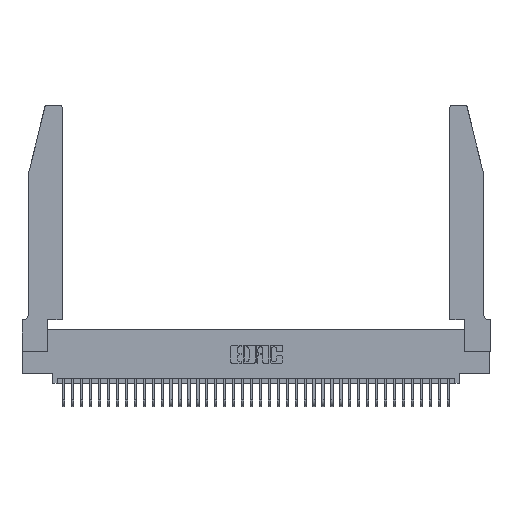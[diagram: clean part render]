
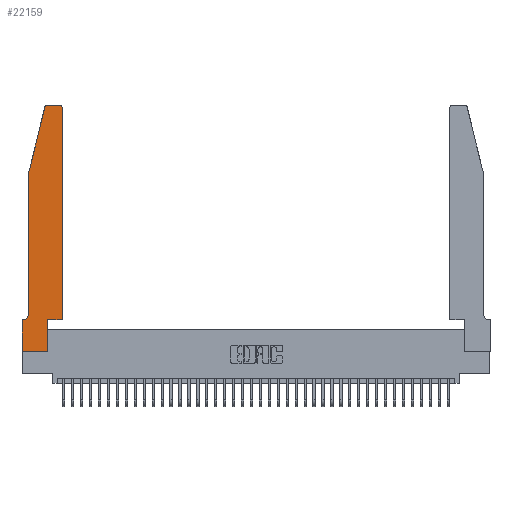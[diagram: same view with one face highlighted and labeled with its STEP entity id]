
A CAD part, top view. The second image highlights one B-rep face of the part: STEP entity #22159.
In plain terms, the highlighted planar face has unit normal (0, 0, 1).
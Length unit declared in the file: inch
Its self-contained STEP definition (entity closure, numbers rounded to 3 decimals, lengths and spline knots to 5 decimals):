
#625 = EDGE_CURVE ( 'NONE', #36127, #12795, #16288, .T. ) ;
#1551 = CARTESIAN_POINT ( 'NONE',  ( 0.4505, 0.35, 0.37 ) ) ;
#2278 = CARTESIAN_POINT ( 'NONE',  ( 0.4505, 2.72, 0.37 ) ) ;
#2791 = CIRCLE ( 'NONE', #31797, 0.03 ) ;
#3465 = EDGE_CURVE ( 'NONE', #24443, #10133, #4185, .T. ) ;
#3854 = CARTESIAN_POINT ( 'NONE',  ( 0., 0.35, 0.37 ) ) ;
#4185 = LINE ( 'NONE', #26175, #34276 ) ;
#4391 = VERTEX_POINT ( 'NONE', #27126 ) ;
#4457 = CARTESIAN_POINT ( 'NONE',  ( 0.4505, 0.35, 0.37 ) ) ;
#4560 = DIRECTION ( 'NONE',  ( 0., 1., 0. ) ) ;
#5130 = CARTESIAN_POINT ( 'NONE',  ( 0.4505, 0.35, 0.37 ) ) ;
#5226 = PLANE ( 'NONE',  #8894 ) ;
#5331 = VECTOR ( 'NONE', #26125, 39.37008 ) ;
#5971 = VECTOR ( 'NONE', #6633, 39.37008 ) ;
#6633 = DIRECTION ( 'NONE',  ( 0., -1., 0. ) ) ;
#6661 = VECTOR ( 'NONE', #24612, 39.37008 ) ;
#7060 = LINE ( 'NONE', #1551, #21715 ) ;
#7087 = CARTESIAN_POINT ( 'NONE',  ( 0.0055, 0.42, 0.37 ) ) ;
#7164 = CARTESIAN_POINT ( 'NONE',  ( 0.2865, 0.35, 0.37 ) ) ;
#7253 = ORIENTED_EDGE ( 'NONE', *, *, #16335, .T. ) ;
#7454 = VECTOR ( 'NONE', #10865, 39.37008 ) ;
#7785 = VERTEX_POINT ( 'NONE', #35398 ) ;
#8198 = DIRECTION ( 'NONE',  ( 1., 0., 0. ) ) ;
#8477 = CARTESIAN_POINT ( 'NONE',  ( 0.0755, 2., 0.37 ) ) ;
#8894 = AXIS2_PLACEMENT_3D ( 'NONE', #22671, #25734, #8198 ) ;
#8982 = VERTEX_POINT ( 'NONE', #23727 ) ;
#9680 = ORIENTED_EDGE ( 'NONE', *, *, #31655, .T. ) ;
#9687 = CARTESIAN_POINT ( 'NONE',  ( 0.4205, 2.72, 0.37 ) ) ;
#9703 = FACE_OUTER_BOUND ( 'NONE', #21059, .T. ) ;
#10053 = DIRECTION ( 'NONE',  ( -1., 0., 0. ) ) ;
#10133 = VERTEX_POINT ( 'NONE', #14189 ) ;
#10865 = DIRECTION ( 'NONE',  ( 1., 0., 0. ) ) ;
#11170 = ORIENTED_EDGE ( 'NONE', *, *, #29424, .T. ) ;
#11819 = ORIENTED_EDGE ( 'NONE', *, *, #21625, .T. ) ;
#12626 = DIRECTION ( 'NONE',  ( 1., 0., 0. ) ) ;
#12795 = VERTEX_POINT ( 'NONE', #3854 ) ;
#13586 = DIRECTION ( 'NONE',  ( 0., -1., 0. ) ) ;
#13634 = EDGE_CURVE ( 'NONE', #7785, #8982, #29855, .T. ) ;
#14189 = CARTESIAN_POINT ( 'NONE',  ( 0.284, 2.75, 0.37 ) ) ;
#14640 = DIRECTION ( 'NONE',  ( 0., 0., 1. ) ) ;
#15138 = ORIENTED_EDGE ( 'NONE', *, *, #625, .T. ) ;
#15760 = ORIENTED_EDGE ( 'NONE', *, *, #28110, .T. ) ;
#16288 = LINE ( 'NONE', #27148, #6661 ) ;
#16335 = EDGE_CURVE ( 'NONE', #20582, #36127, #30513, .T. ) ;
#16415 = CARTESIAN_POINT ( 'NONE',  ( 0.0755, 2., 0.37 ) ) ;
#17723 = AXIS2_PLACEMENT_3D ( 'NONE', #9687, #30072, #12626 ) ;
#17772 = ORIENTED_EDGE ( 'NONE', *, *, #3465, .T. ) ;
#18530 = CARTESIAN_POINT ( 'NONE',  ( 0.25487, 2.72718, 0.37 ) ) ;
#19223 = EDGE_CURVE ( 'NONE', #20204, #4391, #28672, .T. ) ;
#19450 = EDGE_CURVE ( 'NONE', #8982, #23757, #29118, .T. ) ;
#19528 = VECTOR ( 'NONE', #21244, 39.37008 ) ;
#20204 = VERTEX_POINT ( 'NONE', #18530 ) ;
#20359 = LINE ( 'NONE', #4457, #25387 ) ;
#20582 = VERTEX_POINT ( 'NONE', #23219 ) ;
#20588 = VECTOR ( 'NONE', #13586, 39.37008 ) ;
#20680 = ORIENTED_EDGE ( 'NONE', *, *, #13634, .T. ) ;
#21059 = EDGE_LOOP ( 'NONE', ( #17772, #11819, #21415, #26024, #7253, #15138, #9680, #20680, #24377, #27979, #11170, #15760 ) ) ;
#21244 = DIRECTION ( 'NONE',  ( 0., 1., 0. ) ) ;
#21415 = ORIENTED_EDGE ( 'NONE', *, *, #19223, .T. ) ;
#21625 = EDGE_CURVE ( 'NONE', #10133, #20204, #2791, .T. ) ;
#21715 = VECTOR ( 'NONE', #4560, 39.37008 ) ;
#22159 = ADVANCED_FACE ( 'NONE', ( #9703 ), #5226, .T. ) ;
#22671 = CARTESIAN_POINT ( 'NONE',  ( 0., 0.35, 0.37 ) ) ;
#23219 = CARTESIAN_POINT ( 'NONE',  ( 0.0755, 0.42, 0.37 ) ) ;
#23292 = VERTEX_POINT ( 'NONE', #5130 ) ;
#23396 = LINE ( 'NONE', #35654, #5971 ) ;
#23727 = CARTESIAN_POINT ( 'NONE',  ( 0.2865, 0., 0.37 ) ) ;
#23757 = VERTEX_POINT ( 'NONE', #7164 ) ;
#23807 = EDGE_CURVE ( 'NONE', #23757, #23292, #20359, .T. ) ;
#24377 = ORIENTED_EDGE ( 'NONE', *, *, #19450, .T. ) ;
#24443 = VERTEX_POINT ( 'NONE', #28684 ) ;
#24612 = DIRECTION ( 'NONE',  ( -1., 0., 0. ) ) ;
#24846 = DIRECTION ( 'NONE',  ( 1., 0., 0. ) ) ;
#25387 = VECTOR ( 'NONE', #24846, 39.37008 ) ;
#25464 = CARTESIAN_POINT ( 'NONE',  ( 0., 0., 0.37 ) ) ;
#25734 = DIRECTION ( 'NONE',  ( 0., 0., 1. ) ) ;
#26024 = ORIENTED_EDGE ( 'NONE', *, *, #27011, .T. ) ;
#26125 = DIRECTION ( 'NONE',  ( -0.239, -0.971, 0. ) ) ;
#26175 = CARTESIAN_POINT ( 'NONE',  ( 0.2605, 2.75, 0.37 ) ) ;
#27011 = EDGE_CURVE ( 'NONE', #4391, #20582, #37786, .T. ) ;
#27126 = CARTESIAN_POINT ( 'NONE',  ( 0.0755, 2., 0.37 ) ) ;
#27148 = CARTESIAN_POINT ( 'NONE',  ( 0.0755, 0.35, 0.37 ) ) ;
#27561 = DIRECTION ( 'NONE',  ( 0., 0., -1. ) ) ;
#27979 = ORIENTED_EDGE ( 'NONE', *, *, #23807, .T. ) ;
#28110 = EDGE_CURVE ( 'NONE', #32498, #24443, #34508, .T. ) ;
#28672 = LINE ( 'NONE', #8477, #5331 ) ;
#28684 = CARTESIAN_POINT ( 'NONE',  ( 0.4205, 2.75, 0.37 ) ) ;
#29086 = DIRECTION ( 'NONE',  ( -1., 0., 0. ) ) ;
#29118 = LINE ( 'NONE', #35663, #19528 ) ;
#29424 = EDGE_CURVE ( 'NONE', #23292, #32498, #7060, .T. ) ;
#29855 = LINE ( 'NONE', #25464, #7454 ) ;
#30072 = DIRECTION ( 'NONE',  ( 0., 0., 1. ) ) ;
#30513 = CIRCLE ( 'NONE', #37517, 0.07 ) ;
#31655 = EDGE_CURVE ( 'NONE', #12795, #7785, #23396, .T. ) ;
#31797 = AXIS2_PLACEMENT_3D ( 'NONE', #32048, #14640, #34942 ) ;
#32048 = CARTESIAN_POINT ( 'NONE',  ( 0.284, 2.72, 0.37 ) ) ;
#32498 = VERTEX_POINT ( 'NONE', #2278 ) ;
#34276 = VECTOR ( 'NONE', #29086, 39.37008 ) ;
#34508 = CIRCLE ( 'NONE', #17723, 0.03 ) ;
#34561 = CARTESIAN_POINT ( 'NONE',  ( 0.0055, 0.35, 0.37 ) ) ;
#34942 = DIRECTION ( 'NONE',  ( 1., 0., 0. ) ) ;
#35398 = CARTESIAN_POINT ( 'NONE',  ( 0., 0., 0.37 ) ) ;
#35654 = CARTESIAN_POINT ( 'NONE',  ( 0., 0., 0.37 ) ) ;
#35663 = CARTESIAN_POINT ( 'NONE',  ( 0.2865, 0.35, 0.37 ) ) ;
#36127 = VERTEX_POINT ( 'NONE', #34561 ) ;
#37517 = AXIS2_PLACEMENT_3D ( 'NONE', #7087, #27561, #10053 ) ;
#37786 = LINE ( 'NONE', #16415, #20588 ) ;
